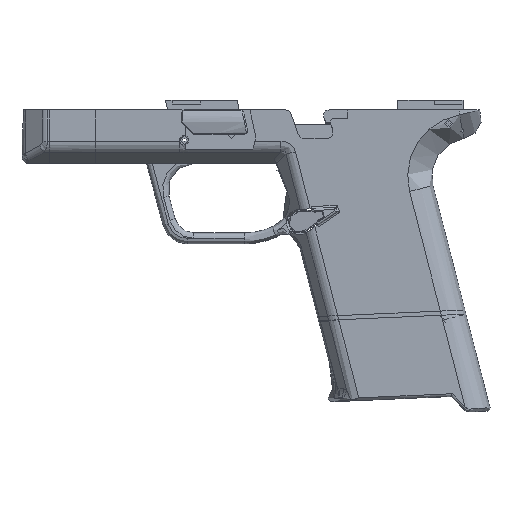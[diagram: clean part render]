
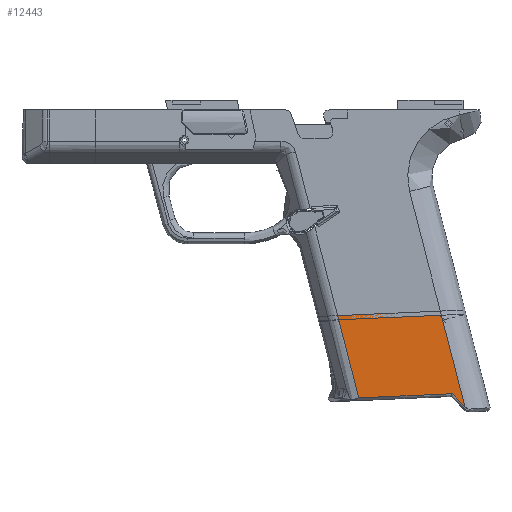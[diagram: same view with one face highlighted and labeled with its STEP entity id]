
A CAD part, left-side view. The second image highlights one B-rep face of the part: STEP entity #12443.
In plain terms, the highlighted face is planar.
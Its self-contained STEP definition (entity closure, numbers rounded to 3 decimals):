
#989=PLANE('',#13636);
#1642=FACE_OUTER_BOUND('',#2359,.T.);
#2359=EDGE_LOOP('',(#11244,#11245,#11246,#11247,#11248));
#3364=LINE('',#23430,#4452);
#3384=LINE('',#24276,#4472);
#3398=LINE('',#24697,#4486);
#3399=LINE('',#24701,#4487);
#3400=LINE('',#24702,#4488);
#4452=VECTOR('',#16564,10.);
#4472=VECTOR('',#16656,10.);
#4486=VECTOR('',#16728,10.);
#4487=VECTOR('',#16733,10.);
#4488=VECTOR('',#16734,10.);
#5934=VERTEX_POINT('',#23408);
#5936=VERTEX_POINT('',#23428);
#5990=VERTEX_POINT('',#24275);
#6009=VERTEX_POINT('',#24538);
#6017=VERTEX_POINT('',#24700);
#7658=EDGE_CURVE('',#5936,#5934,#3364,.T.);
#7740=EDGE_CURVE('',#5990,#5934,#3384,.T.);
#7785=EDGE_CURVE('',#6009,#5936,#3398,.T.);
#7786=EDGE_CURVE('',#6017,#6009,#3399,.T.);
#7787=EDGE_CURVE('',#6017,#5990,#3400,.T.);
#11244=ORIENTED_EDGE('',*,*,#7658,.F.);
#11245=ORIENTED_EDGE('',*,*,#7785,.F.);
#11246=ORIENTED_EDGE('',*,*,#7786,.F.);
#11247=ORIENTED_EDGE('',*,*,#7787,.T.);
#11248=ORIENTED_EDGE('',*,*,#7740,.T.);
#12443=ADVANCED_FACE('',(#1642),#989,.T.);
#13636=AXIS2_PLACEMENT_3D('',#24699,#16731,#16732);
#16564=DIRECTION('',(0.,0.999,0.044));
#16656=DIRECTION('',(0.,-0.249,0.969));
#16728=DIRECTION('',(0.,0.697,-0.717));
#16731=DIRECTION('center_axis',(1.,0.,0.));
#16732=DIRECTION('ref_axis',(0.,0.999,0.044));
#16733=DIRECTION('',(0.,-0.249,0.969));
#16734=DIRECTION('',(0.,0.999,0.044));
#23408=CARTESIAN_POINT('',(22.175,-44.727,96.906));
#23428=CARTESIAN_POINT('',(22.175,-78.67,95.402));
#23430=CARTESIAN_POINT('',(22.175,-44.598,96.911));
#24275=CARTESIAN_POINT('',(22.175,-37.062,67.087));
#24276=CARTESIAN_POINT('',(22.175,-37.062,67.087));
#24538=CARTESIAN_POINT('',(22.175,-83.249,100.107));
#24697=CARTESIAN_POINT('',(22.175,-73.025,89.603));
#24699=CARTESIAN_POINT('Origin',(22.175,-74.337,65.435));
#24700=CARTESIAN_POINT('',(22.175,-74.337,65.435));
#24701=CARTESIAN_POINT('',(22.175,-74.337,65.435));
#24702=CARTESIAN_POINT('',(22.175,-40.4,66.939));
